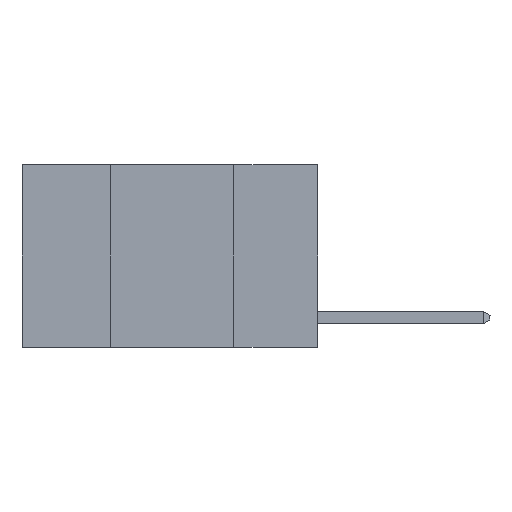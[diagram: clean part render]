
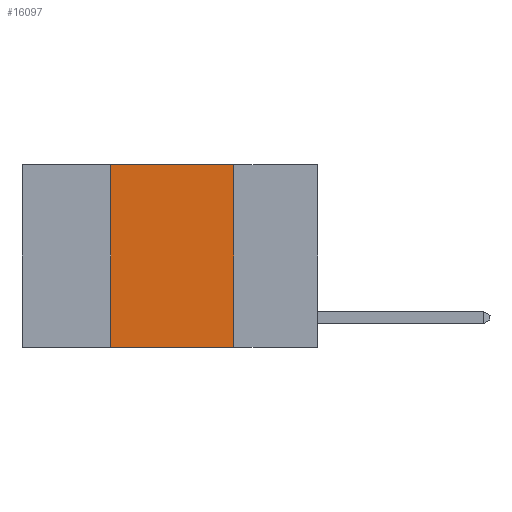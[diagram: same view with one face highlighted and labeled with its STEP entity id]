
A CAD part, left-side view. The second image highlights one B-rep face of the part: STEP entity #16097.
In plain terms, the highlighted planar face has unit normal (-1, 0, 0).
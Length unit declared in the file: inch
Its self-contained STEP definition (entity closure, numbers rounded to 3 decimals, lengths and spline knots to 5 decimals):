
#261 = DIRECTION ( 'NONE',  ( 0., -1., 0. ) ) ;
#361 = CARTESIAN_POINT ( 'NONE',  ( 0., 0.17, -0.37 ) ) ;
#1267 = VERTEX_POINT ( 'NONE', #7788 ) ;
#1454 = LINE ( 'NONE', #14307, #11725 ) ;
#1805 = PLANE ( 'NONE',  #8398 ) ;
#1850 = EDGE_CURVE ( 'NONE', #13706, #5182, #18024, .T. ) ;
#2113 = CARTESIAN_POINT ( 'NONE',  ( 0., 0.17, 0. ) ) ;
#2240 = CARTESIAN_POINT ( 'NONE',  ( 0., 0.42, 0. ) ) ;
#3034 = EDGE_CURVE ( 'NONE', #15929, #1267, #5316, .T. ) ;
#3390 = ORIENTED_EDGE ( 'NONE', *, *, #1850, .F. ) ;
#5182 = VERTEX_POINT ( 'NONE', #361 ) ;
#5316 = LINE ( 'NONE', #2240, #12734 ) ;
#5346 = ORIENTED_EDGE ( 'NONE', *, *, #14640, .T. ) ;
#6056 = DIRECTION ( 'NONE',  ( 0., 0., -1. ) ) ;
#6129 = FACE_OUTER_BOUND ( 'NONE', #16069, .T. ) ;
#6359 = EDGE_CURVE ( 'NONE', #1267, #13706, #1454, .T. ) ;
#7573 = DIRECTION ( 'NONE',  ( 0., 0., -1. ) ) ;
#7788 = CARTESIAN_POINT ( 'NONE',  ( 0., 0.42, 0. ) ) ;
#8398 = AXIS2_PLACEMENT_3D ( 'NONE', #11576, #14399, #6056 ) ;
#8504 = CARTESIAN_POINT ( 'NONE',  ( 0., 0.42, -0.37 ) ) ;
#8957 = CARTESIAN_POINT ( 'NONE',  ( 0., 0.17, 0. ) ) ;
#10603 = VECTOR ( 'NONE', #7573, 39.37008 ) ;
#11576 = CARTESIAN_POINT ( 'NONE',  ( 0., 0.6, 0. ) ) ;
#11611 = VECTOR ( 'NONE', #12505, 39.37008 ) ;
#11725 = VECTOR ( 'NONE', #261, 39.37008 ) ;
#11912 = ORIENTED_EDGE ( 'NONE', *, *, #3034, .F. ) ;
#12019 = DIRECTION ( 'NONE',  ( 0., 0., 1. ) ) ;
#12505 = DIRECTION ( 'NONE',  ( 0., -1., 0. ) ) ;
#12734 = VECTOR ( 'NONE', #12019, 39.37008 ) ;
#13050 = ORIENTED_EDGE ( 'NONE', *, *, #6359, .F. ) ;
#13706 = VERTEX_POINT ( 'NONE', #2113 ) ;
#14307 = CARTESIAN_POINT ( 'NONE',  ( 0., 0.6, 0. ) ) ;
#14399 = DIRECTION ( 'NONE',  ( 1., 0., 0. ) ) ;
#14640 = EDGE_CURVE ( 'NONE', #15929, #5182, #15351, .T. ) ;
#15351 = LINE ( 'NONE', #18051, #11611 ) ;
#15929 = VERTEX_POINT ( 'NONE', #8504 ) ;
#16069 = EDGE_LOOP ( 'NONE', ( #3390, #13050, #11912, #5346 ) ) ;
#16097 = ADVANCED_FACE ( 'NONE', ( #6129 ), #1805, .F. ) ;
#18024 = LINE ( 'NONE', #8957, #10603 ) ;
#18051 = CARTESIAN_POINT ( 'NONE',  ( 0., 0.6, -0.37 ) ) ;
